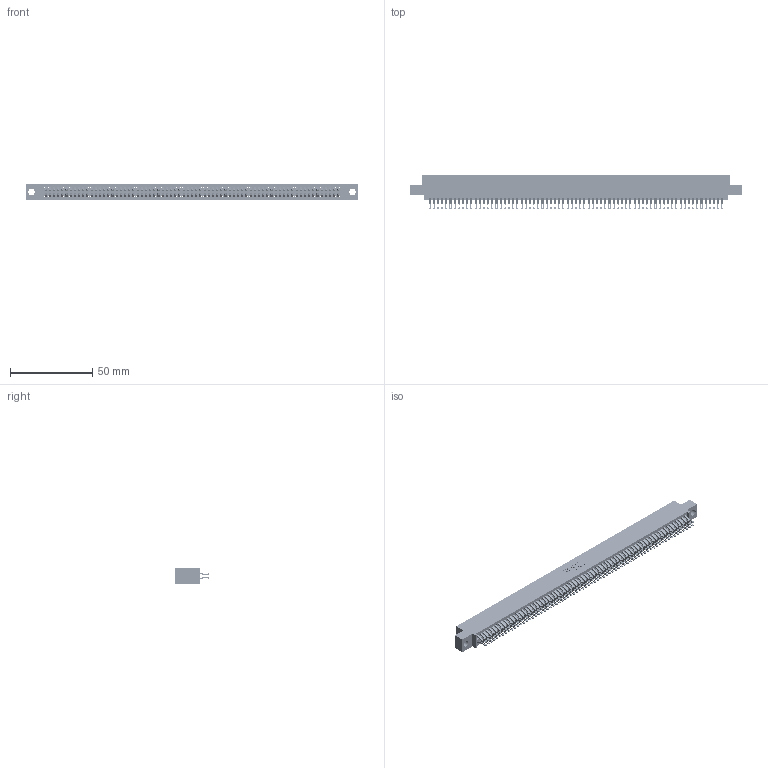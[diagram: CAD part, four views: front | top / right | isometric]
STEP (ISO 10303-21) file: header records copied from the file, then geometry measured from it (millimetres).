
FILE_DESCRIPTION (( 'STEP AP203' ), '1' );
FILE_NAME ('345-142-555-504.STEP', '2018-10-22T13:20:35', ( '' ), ( '' ), 'SwSTEP 2.0', 'SolidWorks 2016', '' );
FILE_SCHEMA (( 'CONFIG_CONTROL_DESIGN' ));
Length unit declared in the file: inch
Products named in the file (3): 345 Part_0.110 Offset - 0.156 Dia-TH; 345-292-001_555 Tail; 345-142-555-504
Assembly tree (143 placements, depth 2):
  345-142-555-504
    345 Part_0.110 Offset - 0.156 Dia-TH
    345-292-001_555 Tail  x142
Bounding box: 201.55 x 21.13 x 9.4 mm (x, y, z)
Volume: 20098.5 mm3; surface area: 31611.2 mm2
Topology: 143 solids, 143 shells, 8082 faces, 25487 edges, 16990 vertices
Faces by surface type: plane 4486, cylinder 3596
Entity records: 52265 total; most frequent: CARTESIAN_POINT 8770, ORIENTED_EDGE 8674, DIRECTION 7665, EDGE_CURVE 4337, VECTOR 3901, LINE 3901, VERTEX_POINT 2890, AXIS2_PLACEMENT_3D 1882
